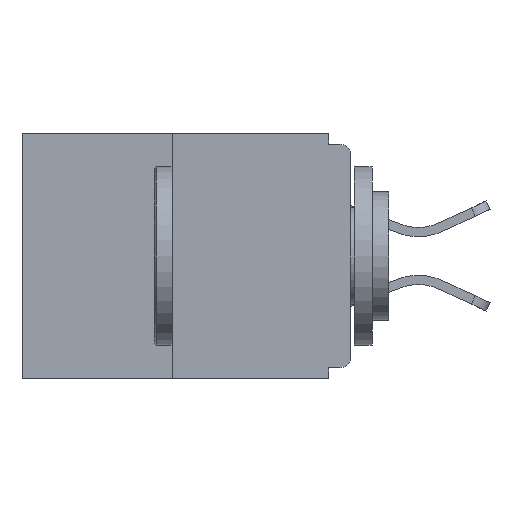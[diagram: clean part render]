
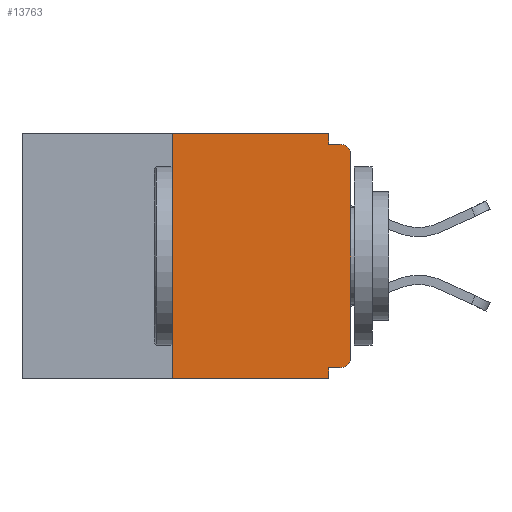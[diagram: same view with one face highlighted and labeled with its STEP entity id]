
A CAD part, left-side view. The second image highlights one B-rep face of the part: STEP entity #13763.
In plain terms, the highlighted planar face has unit normal (-1, 0, 0).
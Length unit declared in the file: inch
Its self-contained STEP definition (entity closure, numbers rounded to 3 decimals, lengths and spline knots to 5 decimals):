
#100 = AXIS2_PLACEMENT_3D ( 'NONE', #1335, #3749, #10478 ) ;
#766 = DIRECTION ( 'NONE',  ( 0., 0., -1. ) ) ;
#903 = LINE ( 'NONE', #8721, #5239 ) ;
#1335 = CARTESIAN_POINT ( 'NONE',  ( 0., 0.015, -0.03 ) ) ;
#1363 = ORIENTED_EDGE ( 'NONE', *, *, #12769, .T. ) ;
#1410 = ORIENTED_EDGE ( 'NONE', *, *, #15286, .F. ) ;
#1412 = VECTOR ( 'NONE', #766, 39.37008 ) ;
#1559 = CARTESIAN_POINT ( 'NONE',  ( 0., 0.031, -0.328 ) ) ;
#1646 = VERTEX_POINT ( 'NONE', #6286 ) ;
#2318 = EDGE_CURVE ( 'NONE', #11291, #2465, #4941, .T. ) ;
#2391 = DIRECTION ( 'NONE',  ( 0., 0., 1. ) ) ;
#2465 = VERTEX_POINT ( 'NONE', #9343 ) ;
#2608 = LINE ( 'NONE', #10536, #12611 ) ;
#2905 = PLANE ( 'NONE',  #15235 ) ;
#3002 = DIRECTION ( 'NONE',  ( 0., 0., -1. ) ) ;
#3322 = CARTESIAN_POINT ( 'NONE',  ( 0., 0.031, -0.343 ) ) ;
#3457 = CARTESIAN_POINT ( 'NONE',  ( 0., 0.031, -0.343 ) ) ;
#3748 = EDGE_CURVE ( 'NONE', #14275, #12657, #16975, .T. ) ;
#3749 = DIRECTION ( 'NONE',  ( -1., 0., 0. ) ) ;
#3935 = CARTESIAN_POINT ( 'NONE',  ( 0., 0.25, 0. ) ) ;
#3982 = EDGE_LOOP ( 'NONE', ( #10276, #4968, #13436, #9034, #4777, #16633, #14926, #1363, #1410, #8086 ) ) ;
#4364 = CARTESIAN_POINT ( 'NONE',  ( 0., 0.015, -0.313 ) ) ;
#4700 = DIRECTION ( 'NONE',  ( 0., -1., 0. ) ) ;
#4777 = ORIENTED_EDGE ( 'NONE', *, *, #11813, .F. ) ;
#4830 = DIRECTION ( 'NONE',  ( 0., 1., 0. ) ) ;
#4930 = CARTESIAN_POINT ( 'NONE',  ( 0., 0.015, -0.015 ) ) ;
#4941 = LINE ( 'NONE', #15104, #15820 ) ;
#4968 = ORIENTED_EDGE ( 'NONE', *, *, #8096, .F. ) ;
#5239 = VECTOR ( 'NONE', #11159, 39.37008 ) ;
#5548 = FACE_OUTER_BOUND ( 'NONE', #3982, .T. ) ;
#6082 = CARTESIAN_POINT ( 'NONE',  ( 0., 0., -0.328 ) ) ;
#6286 = CARTESIAN_POINT ( 'NONE',  ( 0., 0.25, -0.343 ) ) ;
#6498 = DIRECTION ( 'NONE',  ( 0., 0., -1. ) ) ;
#6567 = CARTESIAN_POINT ( 'NONE',  ( 0., 0.031, 0. ) ) ;
#7297 = CARTESIAN_POINT ( 'NONE',  ( 0., 0., -0.03 ) ) ;
#7723 = VECTOR ( 'NONE', #6498, 39.37008 ) ;
#8086 = ORIENTED_EDGE ( 'NONE', *, *, #9448, .F. ) ;
#8096 = EDGE_CURVE ( 'NONE', #1646, #11291, #9643, .T. ) ;
#8285 = LINE ( 'NONE', #6082, #14842 ) ;
#8466 = VERTEX_POINT ( 'NONE', #8742 ) ;
#8721 = CARTESIAN_POINT ( 'NONE',  ( 0., 0., -0.015 ) ) ;
#8742 = CARTESIAN_POINT ( 'NONE',  ( 0., 0., -0.313 ) ) ;
#8919 = CARTESIAN_POINT ( 'NONE',  ( 0., 0.015, -0.328 ) ) ;
#9034 = ORIENTED_EDGE ( 'NONE', *, *, #3748, .F. ) ;
#9100 = CARTESIAN_POINT ( 'NONE',  ( 0., 0.25, 0. ) ) ;
#9343 = CARTESIAN_POINT ( 'NONE',  ( 0., 0.031, 0. ) ) ;
#9448 = EDGE_CURVE ( 'NONE', #2465, #15126, #12226, .T. ) ;
#9492 = DIRECTION ( 'NONE',  ( 1., 0., 0. ) ) ;
#9523 = VECTOR ( 'NONE', #11645, 39.37008 ) ;
#9579 = CIRCLE ( 'NONE', #11994, 0.015 ) ;
#9643 = LINE ( 'NONE', #9100, #15345 ) ;
#10276 = ORIENTED_EDGE ( 'NONE', *, *, #2318, .F. ) ;
#10478 = DIRECTION ( 'NONE',  ( 0., 0., -1. ) ) ;
#10536 = CARTESIAN_POINT ( 'NONE',  ( 0., 0., 0. ) ) ;
#10786 = DIRECTION ( 'NONE',  ( -1., 0., 0. ) ) ;
#10930 = DIRECTION ( 'NONE',  ( 0., 0., -1. ) ) ;
#11159 = DIRECTION ( 'NONE',  ( 0., -1., 0. ) ) ;
#11291 = VERTEX_POINT ( 'NONE', #3935 ) ;
#11645 = DIRECTION ( 'NONE',  ( 0., -1., 0. ) ) ;
#11651 = DIRECTION ( 'NONE',  ( 0., 0., 1. ) ) ;
#11813 = EDGE_CURVE ( 'NONE', #14747, #14275, #8285, .T. ) ;
#11994 = AXIS2_PLACEMENT_3D ( 'NONE', #4364, #10786, #3002 ) ;
#12226 = LINE ( 'NONE', #6567, #7723 ) ;
#12611 = VECTOR ( 'NONE', #2391, 39.37008 ) ;
#12657 = VERTEX_POINT ( 'NONE', #3322 ) ;
#12769 = EDGE_CURVE ( 'NONE', #16737, #15395, #13372, .T. ) ;
#13199 = LINE ( 'NONE', #16881, #9523 ) ;
#13372 = CIRCLE ( 'NONE', #100, 0.015 ) ;
#13422 = CARTESIAN_POINT ( 'NONE',  ( 0., 0.46, 0. ) ) ;
#13436 = ORIENTED_EDGE ( 'NONE', *, *, #16020, .T. ) ;
#13763 = ADVANCED_FACE ( 'NONE', ( #5548 ), #2905, .F. ) ;
#14275 = VERTEX_POINT ( 'NONE', #1559 ) ;
#14446 = EDGE_CURVE ( 'NONE', #14747, #8466, #9579, .T. ) ;
#14462 = EDGE_CURVE ( 'NONE', #8466, #16737, #2608, .T. ) ;
#14747 = VERTEX_POINT ( 'NONE', #8919 ) ;
#14842 = VECTOR ( 'NONE', #4830, 39.37008 ) ;
#14926 = ORIENTED_EDGE ( 'NONE', *, *, #14462, .T. ) ;
#15104 = CARTESIAN_POINT ( 'NONE',  ( 0., 0.46, 0. ) ) ;
#15115 = CARTESIAN_POINT ( 'NONE',  ( 0., 0.031, -0.015 ) ) ;
#15126 = VERTEX_POINT ( 'NONE', #15115 ) ;
#15235 = AXIS2_PLACEMENT_3D ( 'NONE', #13422, #9492, #10930 ) ;
#15286 = EDGE_CURVE ( 'NONE', #15126, #15395, #903, .T. ) ;
#15345 = VECTOR ( 'NONE', #11651, 39.37008 ) ;
#15395 = VERTEX_POINT ( 'NONE', #4930 ) ;
#15820 = VECTOR ( 'NONE', #4700, 39.37008 ) ;
#16020 = EDGE_CURVE ( 'NONE', #1646, #12657, #13199, .T. ) ;
#16633 = ORIENTED_EDGE ( 'NONE', *, *, #14446, .T. ) ;
#16737 = VERTEX_POINT ( 'NONE', #7297 ) ;
#16881 = CARTESIAN_POINT ( 'NONE',  ( 0., 0.46, -0.343 ) ) ;
#16975 = LINE ( 'NONE', #3457, #1412 ) ;
